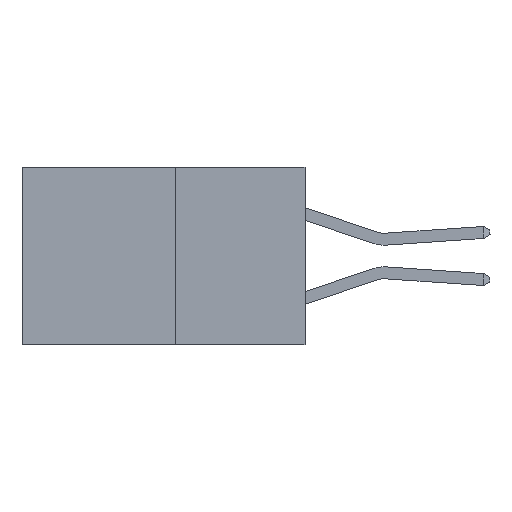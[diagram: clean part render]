
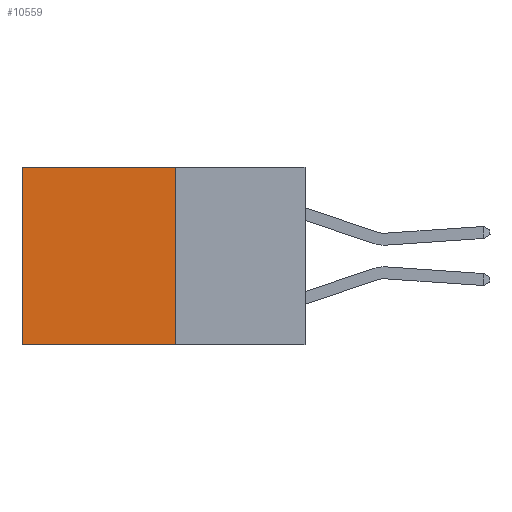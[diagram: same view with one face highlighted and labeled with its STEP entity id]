
A CAD part, left-side view. The second image highlights one B-rep face of the part: STEP entity #10559.
In plain terms, the highlighted planar face has unit normal (-1, 0, 0).
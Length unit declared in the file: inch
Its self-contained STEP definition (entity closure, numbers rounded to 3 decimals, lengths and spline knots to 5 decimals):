
#2300 = VERTEX_POINT ( 'NONE', #3416 ) ;
#2566 = PLANE ( 'NONE',  #21372 ) ;
#3349 = ORIENTED_EDGE ( 'NONE', *, *, #4360, .F. ) ;
#3416 = CARTESIAN_POINT ( 'NONE',  ( 0.277, 0.27, 0. ) ) ;
#3619 = CARTESIAN_POINT ( 'NONE',  ( 0.277, 0.27, -0.37 ) ) ;
#3684 = DIRECTION ( 'NONE',  ( 0., 0., -1. ) ) ;
#3712 = DIRECTION ( 'NONE',  ( 0., 1., 0. ) ) ;
#4039 = CARTESIAN_POINT ( 'NONE',  ( 0.277, 0.27, -0.37 ) ) ;
#4360 = EDGE_CURVE ( 'NONE', #6745, #9455, #12984, .T. ) ;
#4404 = EDGE_LOOP ( 'NONE', ( #15557, #3349, #11873, #10884 ) ) ;
#4541 = DIRECTION ( 'NONE',  ( 0., 0., -1. ) ) ;
#4566 = DIRECTION ( 'NONE',  ( 1., 0., 0. ) ) ;
#5900 = VECTOR ( 'NONE', #3684, 39.37008 ) ;
#6745 = VERTEX_POINT ( 'NONE', #4039 ) ;
#7869 = VECTOR ( 'NONE', #3712, 39.37008 ) ;
#8989 = EDGE_CURVE ( 'NONE', #2300, #6745, #21261, .T. ) ;
#9455 = VERTEX_POINT ( 'NONE', #22654 ) ;
#10559 = ADVANCED_FACE ( 'NONE', ( #15189 ), #2566, .F. ) ;
#10884 = ORIENTED_EDGE ( 'NONE', *, *, #20865, .T. ) ;
#11459 = CARTESIAN_POINT ( 'NONE',  ( 0.277, 0.27, -0.37 ) ) ;
#11873 = ORIENTED_EDGE ( 'NONE', *, *, #8989, .F. ) ;
#12323 = EDGE_CURVE ( 'NONE', #14690, #9455, #22912, .T. ) ;
#12634 = CARTESIAN_POINT ( 'NONE',  ( 0.277, 0.27, 0. ) ) ;
#12984 = LINE ( 'NONE', #3619, #7869 ) ;
#14257 = CARTESIAN_POINT ( 'NONE',  ( 0.277, 0.27, -0.37 ) ) ;
#14690 = VERTEX_POINT ( 'NONE', #18292 ) ;
#14803 = LINE ( 'NONE', #12634, #19908 ) ;
#15189 = FACE_OUTER_BOUND ( 'NONE', #4404, .T. ) ;
#15557 = ORIENTED_EDGE ( 'NONE', *, *, #12323, .T. ) ;
#16400 = DIRECTION ( 'NONE',  ( 0., 1., 0. ) ) ;
#17245 = VECTOR ( 'NONE', #4541, 39.37008 ) ;
#18104 = DIRECTION ( 'NONE',  ( 0., 0., -1. ) ) ;
#18292 = CARTESIAN_POINT ( 'NONE',  ( 0.277, 0.59, 0. ) ) ;
#19908 = VECTOR ( 'NONE', #16400, 39.37008 ) ;
#20865 = EDGE_CURVE ( 'NONE', #2300, #14690, #14803, .T. ) ;
#21261 = LINE ( 'NONE', #11459, #5900 ) ;
#21372 = AXIS2_PLACEMENT_3D ( 'NONE', #14257, #4566, #18104 ) ;
#21923 = CARTESIAN_POINT ( 'NONE',  ( 0.277, 0.59, -0.37 ) ) ;
#22654 = CARTESIAN_POINT ( 'NONE',  ( 0.277, 0.59, -0.37 ) ) ;
#22912 = LINE ( 'NONE', #21923, #17245 ) ;
